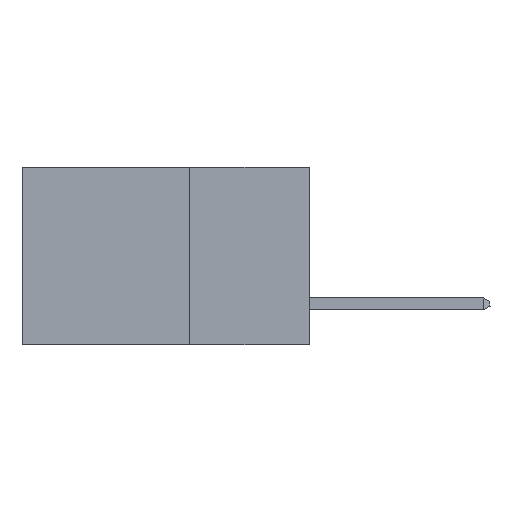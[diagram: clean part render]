
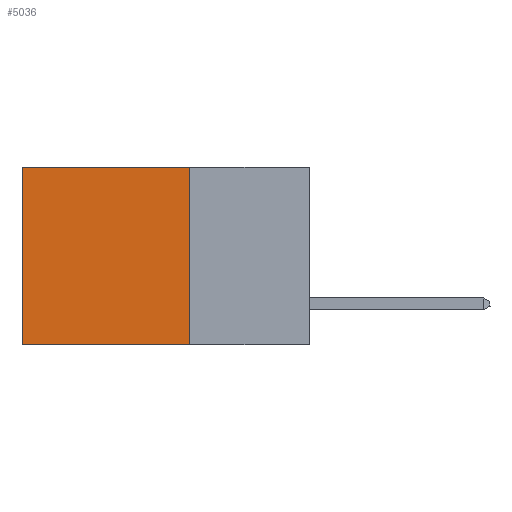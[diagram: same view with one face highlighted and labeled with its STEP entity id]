
A CAD part, left-side view. The second image highlights one B-rep face of the part: STEP entity #5036.
In plain terms, the highlighted planar face has unit normal (-1, 0, 0).
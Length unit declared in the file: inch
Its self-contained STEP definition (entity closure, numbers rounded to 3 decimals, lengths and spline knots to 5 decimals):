
#608 = ORIENTED_EDGE ( 'NONE', *, *, #17824, .T. ) ;
#1082 = LINE ( 'NONE', #5578, #10561 ) ;
#1170 = LINE ( 'NONE', #17152, #21918 ) ;
#3585 = CARTESIAN_POINT ( 'NONE',  ( 0.2875, 0.6, -0.37 ) ) ;
#3804 = VECTOR ( 'NONE', #25418, 39.37008 ) ;
#4792 = CARTESIAN_POINT ( 'NONE',  ( 0.2875, 0.25, 0. ) ) ;
#5036 = ADVANCED_FACE ( 'NONE', ( #22665 ), #19073, .F. ) ;
#5405 = VERTEX_POINT ( 'NONE', #4792 ) ;
#5578 = CARTESIAN_POINT ( 'NONE',  ( 0.2875, 0.25, 0. ) ) ;
#6169 = VERTEX_POINT ( 'NONE', #3585 ) ;
#7048 = CARTESIAN_POINT ( 'NONE',  ( 0.2875, 0.25, 0. ) ) ;
#7558 = ORIENTED_EDGE ( 'NONE', *, *, #10537, .T. ) ;
#8481 = LINE ( 'NONE', #23041, #13513 ) ;
#9028 = CARTESIAN_POINT ( 'NONE',  ( 0.2875, 0.6, 0. ) ) ;
#10210 = ORIENTED_EDGE ( 'NONE', *, *, #13093, .F. ) ;
#10537 = EDGE_CURVE ( 'NONE', #15955, #6169, #11070, .T. ) ;
#10561 = VECTOR ( 'NONE', #19609, 39.37008 ) ;
#10954 = DIRECTION ( 'NONE',  ( 0., 0., -1. ) ) ;
#11070 = LINE ( 'NONE', #23401, #3804 ) ;
#11222 = AXIS2_PLACEMENT_3D ( 'NONE', #7048, #23328, #10954 ) ;
#11919 = VERTEX_POINT ( 'NONE', #16694 ) ;
#12528 = EDGE_LOOP ( 'NONE', ( #7558, #22061, #10210, #608 ) ) ;
#13093 = EDGE_CURVE ( 'NONE', #5405, #11919, #1082, .T. ) ;
#13513 = VECTOR ( 'NONE', #20270, 39.37008 ) ;
#15955 = VERTEX_POINT ( 'NONE', #9028 ) ;
#16420 = EDGE_CURVE ( 'NONE', #11919, #6169, #8481, .T. ) ;
#16694 = CARTESIAN_POINT ( 'NONE',  ( 0.2875, 0.25, -0.37 ) ) ;
#17152 = CARTESIAN_POINT ( 'NONE',  ( 0.2875, 0.25, 0. ) ) ;
#17824 = EDGE_CURVE ( 'NONE', #5405, #15955, #1170, .T. ) ;
#19073 = PLANE ( 'NONE',  #11222 ) ;
#19609 = DIRECTION ( 'NONE',  ( 0., 0., -1. ) ) ;
#20270 = DIRECTION ( 'NONE',  ( 0., 1., 0. ) ) ;
#21315 = DIRECTION ( 'NONE',  ( 0., 1., 0. ) ) ;
#21918 = VECTOR ( 'NONE', #21315, 39.37008 ) ;
#22061 = ORIENTED_EDGE ( 'NONE', *, *, #16420, .F. ) ;
#22665 = FACE_OUTER_BOUND ( 'NONE', #12528, .T. ) ;
#23041 = CARTESIAN_POINT ( 'NONE',  ( 0.2875, 0.25, -0.37 ) ) ;
#23328 = DIRECTION ( 'NONE',  ( 1., 0., 0. ) ) ;
#23401 = CARTESIAN_POINT ( 'NONE',  ( 0.2875, 0.6, 0. ) ) ;
#25418 = DIRECTION ( 'NONE',  ( 0., 0., -1. ) ) ;
